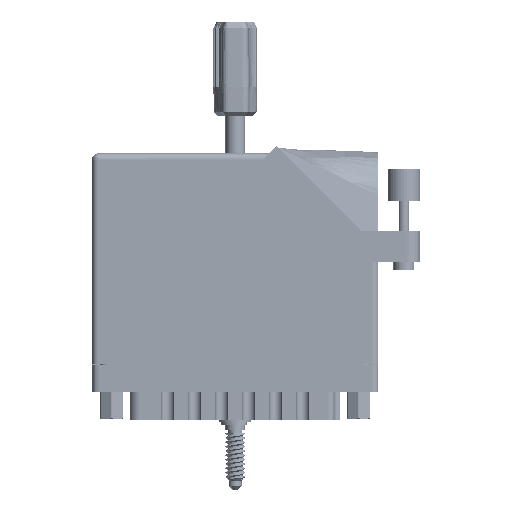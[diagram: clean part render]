
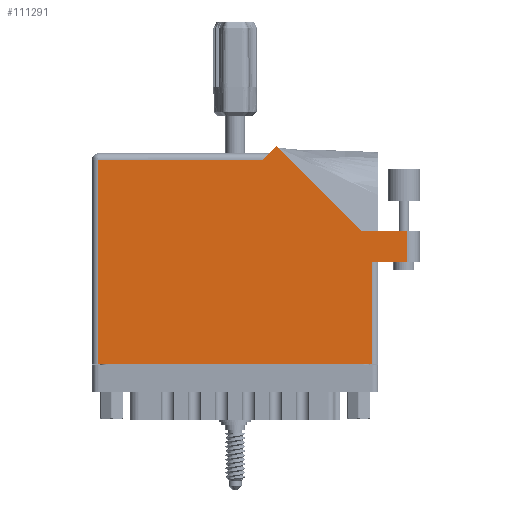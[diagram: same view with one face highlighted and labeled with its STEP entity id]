
A CAD part, front view. The second image highlights one B-rep face of the part: STEP entity #111291.
In plain terms, the highlighted face is planar.
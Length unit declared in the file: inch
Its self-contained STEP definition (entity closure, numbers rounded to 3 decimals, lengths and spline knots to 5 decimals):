
#339 = ORIENTED_EDGE ( 'NONE', *, *, #32207, .T. ) ;
#777 = ORIENTED_EDGE ( 'NONE', *, *, #39261, .T. ) ;
#2991 = VECTOR ( 'NONE', #25574, 39.37008 ) ;
#3272 = CARTESIAN_POINT ( 'NONE',  ( 1.643, 1.968, 0. ) ) ;
#6961 = CARTESIAN_POINT ( 'NONE',  ( 3.03, 0.98, 0. ) ) ;
#7012 = ORIENTED_EDGE ( 'NONE', *, *, #19329, .T. ) ;
#8195 = CARTESIAN_POINT ( 'NONE',  ( 2.58942, 1.287, 0. ) ) ;
#10887 = EDGE_CURVE ( 'NONE', #47657, #11763, #72850, .T. ) ;
#11585 = FACE_OUTER_BOUND ( 'NONE', #104183, .T. ) ;
#11763 = VERTEX_POINT ( 'NONE', #115770 ) ;
#14002 = VECTOR ( 'NONE', #108890, 39.37008 ) ;
#14750 = DIRECTION ( 'NONE',  ( 0., -1., 0. ) ) ;
#14935 = CARTESIAN_POINT ( 'NONE',  ( 0.062, 1.968, 0. ) ) ;
#15327 = CARTESIAN_POINT ( 'NONE',  ( 2.693, 0.98, 0. ) ) ;
#17180 = AXIS2_PLACEMENT_3D ( 'NONE', #94274, #58111, #103099 ) ;
#19329 = EDGE_CURVE ( 'NONE', #33538, #105602, #107336, .T. ) ;
#20968 = VECTOR ( 'NONE', #44568, 39.37008 ) ;
#23694 = VERTEX_POINT ( 'NONE', #99602 ) ;
#25574 = DIRECTION ( 'NONE',  ( 0., 1., 0. ) ) ;
#31809 = ORIENTED_EDGE ( 'NONE', *, *, #85593, .T. ) ;
#32207 = EDGE_CURVE ( 'NONE', #105602, #109406, #85900, .T. ) ;
#33538 = VERTEX_POINT ( 'NONE', #15327 ) ;
#34485 = VECTOR ( 'NONE', #114037, 39.37008 ) ;
#39261 = EDGE_CURVE ( 'NONE', #11763, #110456, #74104, .T. ) ;
#41379 = VECTOR ( 'NONE', #91469, 39.37008 ) ;
#44568 = DIRECTION ( 'NONE',  ( -0.707, -0.707, 0. ) ) ;
#47463 = EDGE_CURVE ( 'NONE', #23694, #52839, #81766, .T. ) ;
#47657 = VERTEX_POINT ( 'NONE', #98070 ) ;
#50853 = CARTESIAN_POINT ( 'NONE',  ( 2.693, 0.98, 0. ) ) ;
#51255 = CARTESIAN_POINT ( 'NONE',  ( 2.693, 0., 0. ) ) ;
#51610 = VECTOR ( 'NONE', #96081, 39.37008 ) ;
#52839 = VERTEX_POINT ( 'NONE', #51255 ) ;
#53381 = CARTESIAN_POINT ( 'NONE',  ( 1.705, 2.03, 0. ) ) ;
#53448 = ORIENTED_EDGE ( 'NONE', *, *, #47463, .T. ) ;
#54304 = CARTESIAN_POINT ( 'NONE',  ( 0., 1.968, 0. ) ) ;
#56226 = VECTOR ( 'NONE', #110102, 39.37008 ) ;
#58004 = EDGE_CURVE ( 'NONE', #52839, #33538, #76312, .T. ) ;
#58111 = DIRECTION ( 'NONE',  ( 0., 0., -1. ) ) ;
#58885 = EDGE_CURVE ( 'NONE', #109406, #47657, #107714, .T. ) ;
#60265 = ORIENTED_EDGE ( 'NONE', *, *, #58004, .T. ) ;
#62735 = VECTOR ( 'NONE', #81731, 39.37008 ) ;
#69365 = CARTESIAN_POINT ( 'NONE',  ( 3.03, 1.287, 0. ) ) ;
#72471 = ORIENTED_EDGE ( 'NONE', *, *, #10887, .T. ) ;
#72850 = LINE ( 'NONE', #8195, #14002 ) ;
#74104 = LINE ( 'NONE', #53381, #20968 ) ;
#76068 = CARTESIAN_POINT ( 'NONE',  ( 0., 0., 0. ) ) ;
#76312 = LINE ( 'NONE', #50853, #2991 ) ;
#81731 = DIRECTION ( 'NONE',  ( 1., 0., 0. ) ) ;
#81766 = LINE ( 'NONE', #76068, #51610 ) ;
#83517 = LINE ( 'NONE', #54304, #56226 ) ;
#84050 = ORIENTED_EDGE ( 'NONE', *, *, #100216, .T. ) ;
#85593 = EDGE_CURVE ( 'NONE', #110456, #115483, #83517, .T. ) ;
#85900 = LINE ( 'NONE', #92252, #41379 ) ;
#89324 = VECTOR ( 'NONE', #14750, 39.37008 ) ;
#91469 = DIRECTION ( 'NONE',  ( 0., 1., 0. ) ) ;
#92252 = CARTESIAN_POINT ( 'NONE',  ( 3.03, 1.287, 0. ) ) ;
#94274 = CARTESIAN_POINT ( 'NONE',  ( 0., 2.03, 0. ) ) ;
#95794 = CARTESIAN_POINT ( 'NONE',  ( 0.062, 0., 0. ) ) ;
#96081 = DIRECTION ( 'NONE',  ( 1., 0., 0. ) ) ;
#98070 = CARTESIAN_POINT ( 'NONE',  ( 2.58942, 1.287, 0. ) ) ;
#99602 = CARTESIAN_POINT ( 'NONE',  ( 0.062, 0., 0. ) ) ;
#100216 = EDGE_CURVE ( 'NONE', #115483, #23694, #103564, .T. ) ;
#103099 = DIRECTION ( 'NONE',  ( -1., 0., 0. ) ) ;
#103564 = LINE ( 'NONE', #95794, #89324 ) ;
#104183 = EDGE_LOOP ( 'NONE', ( #7012, #339, #116959, #72471, #777, #31809, #84050, #53448, #60265 ) ) ;
#104793 = CARTESIAN_POINT ( 'NONE',  ( 3.155, 1.287, 0. ) ) ;
#105602 = VERTEX_POINT ( 'NONE', #6961 ) ;
#107336 = LINE ( 'NONE', #110210, #62735 ) ;
#107714 = LINE ( 'NONE', #104793, #34485 ) ;
#108890 = DIRECTION ( 'NONE',  ( -0.707, 0.707, 0. ) ) ;
#109406 = VERTEX_POINT ( 'NONE', #69365 ) ;
#110102 = DIRECTION ( 'NONE',  ( -1., 0., 0. ) ) ;
#110210 = CARTESIAN_POINT ( 'NONE',  ( 2.755, 0.98, 0. ) ) ;
#110456 = VERTEX_POINT ( 'NONE', #3272 ) ;
#111291 = ADVANCED_FACE ( 'NONE', ( #11585 ), #113138, .F. ) ;
#113138 = PLANE ( 'NONE',  #17180 ) ;
#114037 = DIRECTION ( 'NONE',  ( -1., 0., 0. ) ) ;
#115483 = VERTEX_POINT ( 'NONE', #14935 ) ;
#115770 = CARTESIAN_POINT ( 'NONE',  ( 1.77571, 2.10071, 0. ) ) ;
#116959 = ORIENTED_EDGE ( 'NONE', *, *, #58885, .T. ) ;
